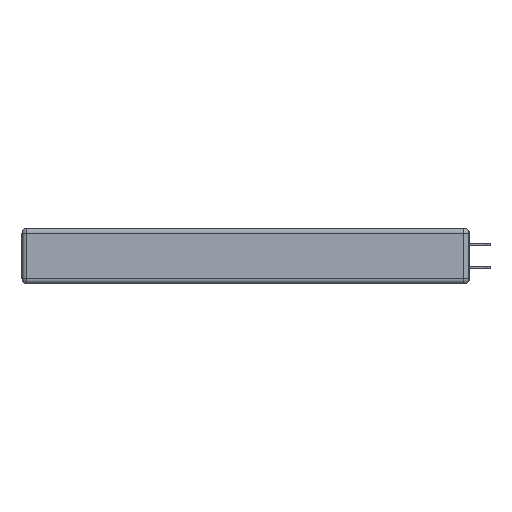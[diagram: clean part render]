
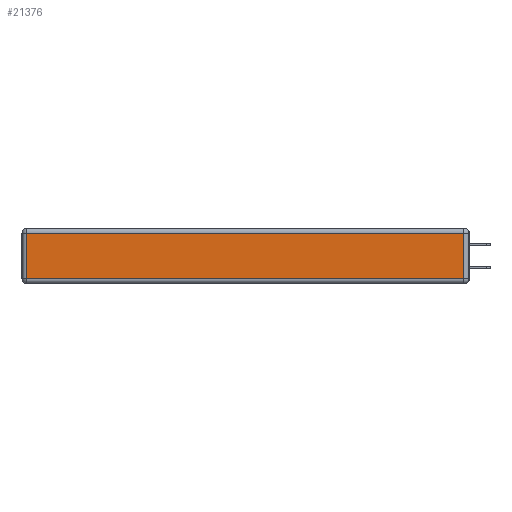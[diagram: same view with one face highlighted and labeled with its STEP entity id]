
A CAD part, left-side view. The second image highlights one B-rep face of the part: STEP entity #21376.
In plain terms, the highlighted planar face has unit normal (-1, 0, 0).
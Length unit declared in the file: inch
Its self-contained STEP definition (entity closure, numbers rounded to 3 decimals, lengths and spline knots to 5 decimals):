
#175 = VERTEX_POINT ( 'NONE', #8024 ) ;
#260 = DIRECTION ( 'NONE',  ( 0., 0., 1. ) ) ;
#2049 = CARTESIAN_POINT ( 'NONE',  ( 0., 2.75, -0.03 ) ) ;
#2502 = DIRECTION ( 'NONE',  ( -1., 0., 0. ) ) ;
#2622 = CARTESIAN_POINT ( 'NONE',  ( 0., 0., -0.313 ) ) ;
#3752 = LINE ( 'NONE', #2622, #16532 ) ;
#3791 = CARTESIAN_POINT ( 'NONE',  ( 0., 2.72, -0.343 ) ) ;
#3865 = EDGE_CURVE ( 'NONE', #24376, #6077, #4737, .T. ) ;
#4737 = LINE ( 'NONE', #3791, #7762 ) ;
#6077 = VERTEX_POINT ( 'NONE', #17171 ) ;
#7139 = DIRECTION ( 'NONE',  ( 0., -1., 0. ) ) ;
#7184 = FACE_OUTER_BOUND ( 'NONE', #24925, .T. ) ;
#7357 = EDGE_CURVE ( 'NONE', #8419, #175, #9254, .T. ) ;
#7762 = VECTOR ( 'NONE', #15149, 39.37008 ) ;
#8024 = CARTESIAN_POINT ( 'NONE',  ( 0., 0.03, -0.03 ) ) ;
#8419 = VERTEX_POINT ( 'NONE', #15742 ) ;
#9254 = LINE ( 'NONE', #14029, #24452 ) ;
#11384 = LINE ( 'NONE', #2049, #12064 ) ;
#12064 = VECTOR ( 'NONE', #19094, 39.37008 ) ;
#14029 = CARTESIAN_POINT ( 'NONE',  ( 0., 0.03, -0.343 ) ) ;
#15149 = DIRECTION ( 'NONE',  ( 0., 0., -1. ) ) ;
#15215 = ORIENTED_EDGE ( 'NONE', *, *, #27356, .T. ) ;
#15742 = CARTESIAN_POINT ( 'NONE',  ( 0., 0.03, -0.313 ) ) ;
#16532 = VECTOR ( 'NONE', #7139, 39.37008 ) ;
#17171 = CARTESIAN_POINT ( 'NONE',  ( 0., 2.72, -0.313 ) ) ;
#17191 = ORIENTED_EDGE ( 'NONE', *, *, #3865, .T. ) ;
#17270 = CARTESIAN_POINT ( 'NONE',  ( 0., 0., -0.343 ) ) ;
#19094 = DIRECTION ( 'NONE',  ( 0., 1., 0. ) ) ;
#19305 = ORIENTED_EDGE ( 'NONE', *, *, #23584, .T. ) ;
#20750 = DIRECTION ( 'NONE',  ( 0., 0., 1. ) ) ;
#21123 = ORIENTED_EDGE ( 'NONE', *, *, #7357, .T. ) ;
#21376 = ADVANCED_FACE ( 'NONE', ( #7184 ), #23549, .T. ) ;
#23549 = PLANE ( 'NONE',  #26970 ) ;
#23584 = EDGE_CURVE ( 'NONE', #6077, #8419, #3752, .T. ) ;
#24376 = VERTEX_POINT ( 'NONE', #27392 ) ;
#24452 = VECTOR ( 'NONE', #20750, 39.37008 ) ;
#24925 = EDGE_LOOP ( 'NONE', ( #19305, #21123, #15215, #17191 ) ) ;
#26970 = AXIS2_PLACEMENT_3D ( 'NONE', #17270, #2502, #260 ) ;
#27356 = EDGE_CURVE ( 'NONE', #175, #24376, #11384, .T. ) ;
#27392 = CARTESIAN_POINT ( 'NONE',  ( 0., 2.72, -0.03 ) ) ;
